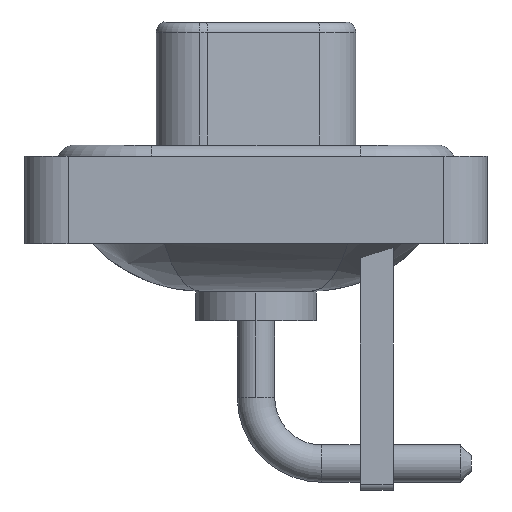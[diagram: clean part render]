
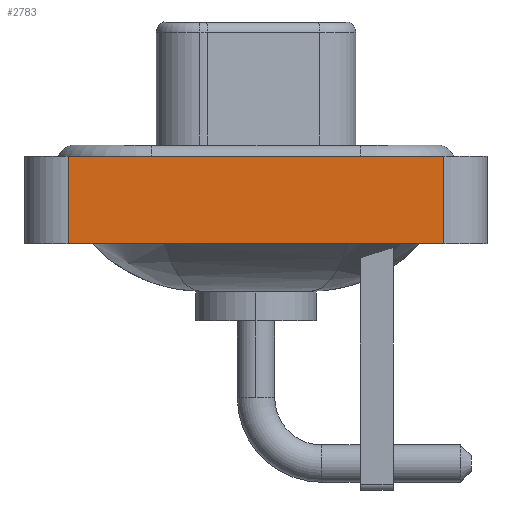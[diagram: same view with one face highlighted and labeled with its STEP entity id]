
A CAD part, left-side view. The second image highlights one B-rep face of the part: STEP entity #2783.
In plain terms, the highlighted planar face has unit normal (-1, 0, 0).
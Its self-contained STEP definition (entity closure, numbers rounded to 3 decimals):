
#1874 = VERTEX_POINT ( 'NONE', #3804 ) ;
#2006 = DIRECTION ( 'NONE',  ( 0., -1., 0. ) ) ;
#2236 = EDGE_CURVE ( 'NONE', #3826, #13486, #4636, .T. ) ;
#2374 = EDGE_LOOP ( 'NONE', ( #15288, #7256, #12946, #5928 ) ) ;
#2783 = ADVANCED_FACE ( 'NONE', ( #4691 ), #4867, .T. ) ;
#3494 = DIRECTION ( 'NONE',  ( 0., 0., 1. ) ) ;
#3804 = CARTESIAN_POINT ( 'NONE',  ( -7.3, -8.55, -3.6 ) ) ;
#3826 = VERTEX_POINT ( 'NONE', #11545 ) ;
#3940 = VECTOR ( 'NONE', #2006, 1000. ) ;
#4454 = DIRECTION ( 'NONE',  ( 0., 0., 1. ) ) ;
#4460 = VECTOR ( 'NONE', #4454, 1000. ) ;
#4636 = LINE ( 'NONE', #4804, #14206 ) ;
#4691 = FACE_OUTER_BOUND ( 'NONE', #2374, .T. ) ;
#4694 = CARTESIAN_POINT ( 'NONE',  ( -7.3, -8.55, 0.4 ) ) ;
#4804 = CARTESIAN_POINT ( 'NONE',  ( -7.3, 8.55, -3.6 ) ) ;
#4867 = PLANE ( 'NONE',  #13660 ) ;
#5928 = ORIENTED_EDGE ( 'NONE', *, *, #8511, .T. ) ;
#6201 = LINE ( 'NONE', #11507, #4460 ) ;
#7256 = ORIENTED_EDGE ( 'NONE', *, *, #12970, .F. ) ;
#8511 = EDGE_CURVE ( 'NONE', #3826, #1874, #10792, .T. ) ;
#8999 = CARTESIAN_POINT ( 'NONE',  ( -7.3, 8.55, 0.4 ) ) ;
#9603 = CARTESIAN_POINT ( 'NONE',  ( -7.3, -8.55, 0.4 ) ) ;
#10792 = LINE ( 'NONE', #12380, #3940 ) ;
#11325 = LINE ( 'NONE', #4694, #16787 ) ;
#11507 = CARTESIAN_POINT ( 'NONE',  ( -7.3, -8.55, -3.6 ) ) ;
#11545 = CARTESIAN_POINT ( 'NONE',  ( -7.3, 8.55, -3.6 ) ) ;
#12380 = CARTESIAN_POINT ( 'NONE',  ( -7.3, -8.55, -3.6 ) ) ;
#12946 = ORIENTED_EDGE ( 'NONE', *, *, #2236, .F. ) ;
#12970 = EDGE_CURVE ( 'NONE', #13486, #13579, #11325, .T. ) ;
#13486 = VERTEX_POINT ( 'NONE', #8999 ) ;
#13579 = VERTEX_POINT ( 'NONE', #9603 ) ;
#13660 = AXIS2_PLACEMENT_3D ( 'NONE', #15519, #15442, #15781 ) ;
#14206 = VECTOR ( 'NONE', #3494, 1000. ) ;
#15288 = ORIENTED_EDGE ( 'NONE', *, *, #15671, .T. ) ;
#15442 = DIRECTION ( 'NONE',  ( -1., 0., 0. ) ) ;
#15519 = CARTESIAN_POINT ( 'NONE',  ( -7.3, -8.55, -3.6 ) ) ;
#15671 = EDGE_CURVE ( 'NONE', #1874, #13579, #6201, .T. ) ;
#15781 = DIRECTION ( 'NONE',  ( 0., 0., 1. ) ) ;
#16663 = DIRECTION ( 'NONE',  ( 0., -1., 0. ) ) ;
#16787 = VECTOR ( 'NONE', #16663, 1000. ) ;
